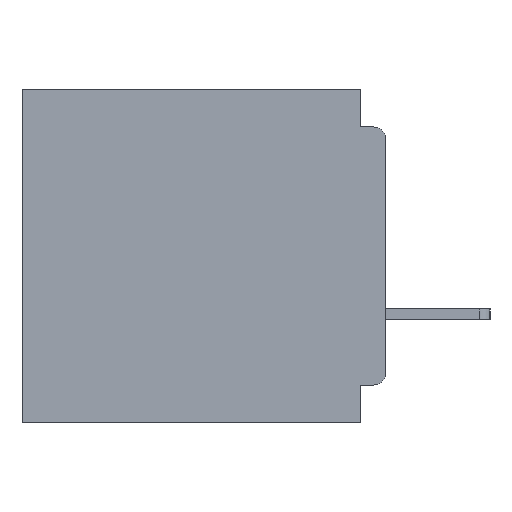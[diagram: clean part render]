
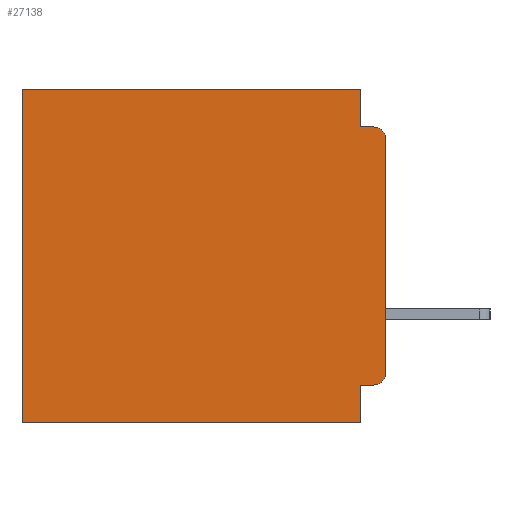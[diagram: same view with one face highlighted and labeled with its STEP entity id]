
A CAD part, left-side view. The second image highlights one B-rep face of the part: STEP entity #27138.
In plain terms, the highlighted planar face has unit normal (-1, 0, 0).
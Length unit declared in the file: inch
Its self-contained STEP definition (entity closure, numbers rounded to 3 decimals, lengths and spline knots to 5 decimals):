
#136 = VERTEX_POINT ( 'NONE', #11055 ) ;
#224 = ORIENTED_EDGE ( 'NONE', *, *, #6671, .F. ) ;
#480 = CIRCLE ( 'NONE', #32783, 0.015 ) ;
#844 = DIRECTION ( 'NONE',  ( 0., 0., -1. ) ) ;
#851 = VERTEX_POINT ( 'NONE', #34279 ) ;
#883 = VECTOR ( 'NONE', #13591, 39.37008 ) ;
#1316 = AXIS2_PLACEMENT_3D ( 'NONE', #13130, #32316, #15931 ) ;
#2450 = DIRECTION ( 'NONE',  ( 0., 1., 0. ) ) ;
#2564 = ORIENTED_EDGE ( 'NONE', *, *, #17320, .F. ) ;
#2639 = CARTESIAN_POINT ( 'NONE',  ( 0.3, 0., -0.4 ) ) ;
#2859 = EDGE_CURVE ( 'NONE', #18395, #136, #30816, .T. ) ;
#3443 = VERTEX_POINT ( 'NONE', #31891 ) ;
#4350 = VECTOR ( 'NONE', #844, 39.37008 ) ;
#4427 = CARTESIAN_POINT ( 'NONE',  ( 0.3, 0., -0.06 ) ) ;
#5442 = CARTESIAN_POINT ( 'NONE',  ( 0.3, 0., -0.4 ) ) ;
#6236 = ORIENTED_EDGE ( 'NONE', *, *, #21732, .T. ) ;
#6671 = EDGE_CURVE ( 'NONE', #22513, #28567, #33403, .T. ) ;
#6888 = CARTESIAN_POINT ( 'NONE',  ( 0.3, 0.031, -0.4 ) ) ;
#6900 = CARTESIAN_POINT ( 'NONE',  ( 0.3, 0., 0. ) ) ;
#7090 = FACE_OUTER_BOUND ( 'NONE', #12698, .T. ) ;
#7372 = VECTOR ( 'NONE', #35599, 39.37008 ) ;
#7622 = ORIENTED_EDGE ( 'NONE', *, *, #19672, .F. ) ;
#8005 = VECTOR ( 'NONE', #14396, 39.37008 ) ;
#8157 = DIRECTION ( 'NONE',  ( 1., 0., 0. ) ) ;
#8961 = AXIS2_PLACEMENT_3D ( 'NONE', #2639, #8157, #27414 ) ;
#9143 = CARTESIAN_POINT ( 'NONE',  ( 0.3, 0.437, -0.4 ) ) ;
#9978 = DIRECTION ( 'NONE',  ( 0., 0., -1. ) ) ;
#10125 = ORIENTED_EDGE ( 'NONE', *, *, #10910, .T. ) ;
#10480 = CARTESIAN_POINT ( 'NONE',  ( 0.3, 0.015, -0.06 ) ) ;
#10499 = CARTESIAN_POINT ( 'NONE',  ( 0.3, 0.031, 0. ) ) ;
#10910 = EDGE_CURVE ( 'NONE', #34915, #851, #20727, .T. ) ;
#11055 = CARTESIAN_POINT ( 'NONE',  ( 0.3, 0.437, 0. ) ) ;
#11653 = LINE ( 'NONE', #28279, #4350 ) ;
#12698 = EDGE_LOOP ( 'NONE', ( #2564, #30328, #23943, #31242, #24587, #6236, #15465, #224, #7622, #10125 ) ) ;
#13117 = LINE ( 'NONE', #29080, #26890 ) ;
#13130 = CARTESIAN_POINT ( 'NONE',  ( 0.3, 0.015, -0.34 ) ) ;
#13266 = DIRECTION ( 'NONE',  ( 0., 0., -1. ) ) ;
#13587 = PLANE ( 'NONE',  #8961 ) ;
#13591 = DIRECTION ( 'NONE',  ( 0., 0., -1. ) ) ;
#14396 = DIRECTION ( 'NONE',  ( 0., 1., 0. ) ) ;
#14490 = CARTESIAN_POINT ( 'NONE',  ( 0.3, 0.015, -0.355 ) ) ;
#15465 = ORIENTED_EDGE ( 'NONE', *, *, #21464, .F. ) ;
#15565 = VERTEX_POINT ( 'NONE', #9143 ) ;
#15589 = LINE ( 'NONE', #5442, #883 ) ;
#15931 = DIRECTION ( 'NONE',  ( 0., 0., -1. ) ) ;
#17320 = EDGE_CURVE ( 'NONE', #20773, #851, #15589, .T. ) ;
#17326 = EDGE_CURVE ( 'NONE', #26398, #3443, #29320, .T. ) ;
#18052 = DIRECTION ( 'NONE',  ( 0., 0., -1. ) ) ;
#18395 = VERTEX_POINT ( 'NONE', #10499 ) ;
#18813 = DIRECTION ( 'NONE',  ( 0., 1., 0. ) ) ;
#18932 = CARTESIAN_POINT ( 'NONE',  ( 0.3, 0., -0.4 ) ) ;
#19161 = CARTESIAN_POINT ( 'NONE',  ( 0.3, 0.031, -0.355 ) ) ;
#19672 = EDGE_CURVE ( 'NONE', #34915, #22513, #30054, .T. ) ;
#20727 = CIRCLE ( 'NONE', #1316, 0.015 ) ;
#20773 = VERTEX_POINT ( 'NONE', #4427 ) ;
#21464 = EDGE_CURVE ( 'NONE', #28567, #15565, #28185, .T. ) ;
#21732 = EDGE_CURVE ( 'NONE', #136, #15565, #13117, .T. ) ;
#21757 = VECTOR ( 'NONE', #2450, 39.37008 ) ;
#22513 = VERTEX_POINT ( 'NONE', #19161 ) ;
#23943 = ORIENTED_EDGE ( 'NONE', *, *, #17326, .F. ) ;
#24587 = ORIENTED_EDGE ( 'NONE', *, *, #2859, .T. ) ;
#26179 = VECTOR ( 'NONE', #9978, 39.37008 ) ;
#26398 = VERTEX_POINT ( 'NONE', #31525 ) ;
#26890 = VECTOR ( 'NONE', #18052, 39.37008 ) ;
#27138 = ADVANCED_FACE ( 'NONE', ( #7090 ), #13587, .F. ) ;
#27414 = DIRECTION ( 'NONE',  ( 0., 0., -1. ) ) ;
#28185 = LINE ( 'NONE', #18932, #21757 ) ;
#28279 = CARTESIAN_POINT ( 'NONE',  ( 0.3, 0.031, 0. ) ) ;
#28567 = VERTEX_POINT ( 'NONE', #6888 ) ;
#29080 = CARTESIAN_POINT ( 'NONE',  ( 0.3, 0.437, -0.4 ) ) ;
#29224 = CARTESIAN_POINT ( 'NONE',  ( 0.3, 0.031, -0.4 ) ) ;
#29320 = LINE ( 'NONE', #32894, #7372 ) ;
#29753 = DIRECTION ( 'NONE',  ( -1., 0., 0. ) ) ;
#29881 = CARTESIAN_POINT ( 'NONE',  ( 0.3, 0., -0.355 ) ) ;
#30054 = LINE ( 'NONE', #29881, #35529 ) ;
#30328 = ORIENTED_EDGE ( 'NONE', *, *, #32635, .T. ) ;
#30816 = LINE ( 'NONE', #6900, #8005 ) ;
#31242 = ORIENTED_EDGE ( 'NONE', *, *, #33044, .F. ) ;
#31525 = CARTESIAN_POINT ( 'NONE',  ( 0.3, 0.031, -0.045 ) ) ;
#31891 = CARTESIAN_POINT ( 'NONE',  ( 0.3, 0.015, -0.045 ) ) ;
#32316 = DIRECTION ( 'NONE',  ( -1., 0., 0. ) ) ;
#32635 = EDGE_CURVE ( 'NONE', #20773, #3443, #480, .T. ) ;
#32783 = AXIS2_PLACEMENT_3D ( 'NONE', #10480, #29753, #13266 ) ;
#32894 = CARTESIAN_POINT ( 'NONE',  ( 0.3, 0., -0.045 ) ) ;
#33044 = EDGE_CURVE ( 'NONE', #18395, #26398, #11653, .T. ) ;
#33403 = LINE ( 'NONE', #29224, #26179 ) ;
#34279 = CARTESIAN_POINT ( 'NONE',  ( 0.3, 0., -0.34 ) ) ;
#34915 = VERTEX_POINT ( 'NONE', #14490 ) ;
#35529 = VECTOR ( 'NONE', #18813, 39.37008 ) ;
#35599 = DIRECTION ( 'NONE',  ( 0., -1., 0. ) ) ;
